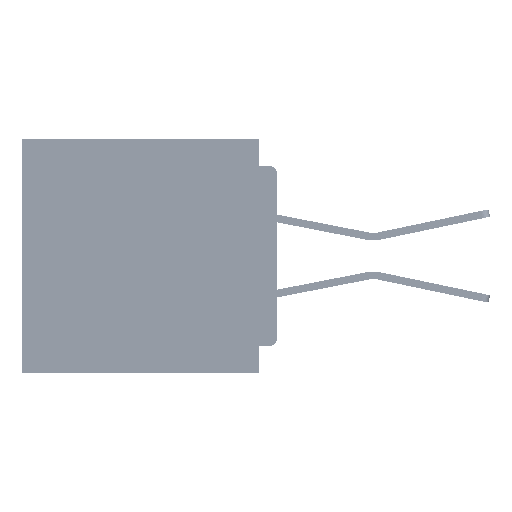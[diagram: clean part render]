
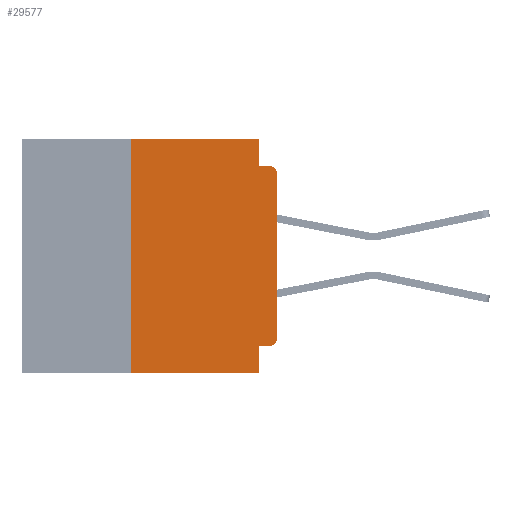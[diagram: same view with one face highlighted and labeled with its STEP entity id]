
A CAD part, left-side view. The second image highlights one B-rep face of the part: STEP entity #29577.
In plain terms, the highlighted planar face has unit normal (-1, 0, 0).
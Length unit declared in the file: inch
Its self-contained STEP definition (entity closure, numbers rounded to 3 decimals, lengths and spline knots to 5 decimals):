
#2946 = VERTEX_POINT ( 'NONE', #14960 ) ;
#3059 = EDGE_CURVE ( 'NONE', #48623, #46420, #39649, .T. ) ;
#3103 = CARTESIAN_POINT ( 'NONE',  ( 0., 0.437, 0. ) ) ;
#4556 = EDGE_CURVE ( 'NONE', #61077, #48860, #14147, .T. ) ;
#5294 = DIRECTION ( 'NONE',  ( 0., 0., -1. ) ) ;
#5375 = CARTESIAN_POINT ( 'NONE',  ( 0., 0.031, 0. ) ) ;
#5551 = VECTOR ( 'NONE', #23703, 39.37008 ) ;
#6043 = EDGE_CURVE ( 'NONE', #21826, #12576, #18952, .T. ) ;
#7128 = EDGE_CURVE ( 'NONE', #57842, #21826, #60957, .T. ) ;
#7191 = VECTOR ( 'NONE', #23229, 39.37008 ) ;
#8165 = CARTESIAN_POINT ( 'NONE',  ( 0., 0.031, -0.355 ) ) ;
#8430 = CARTESIAN_POINT ( 'NONE',  ( 0., 0.015, -0.045 ) ) ;
#8870 = EDGE_CURVE ( 'NONE', #2946, #16719, #47014, .T. ) ;
#9549 = LINE ( 'NONE', #3103, #63035 ) ;
#10191 = ORIENTED_EDGE ( 'NONE', *, *, #39013, .F. ) ;
#10314 = ORIENTED_EDGE ( 'NONE', *, *, #3059, .F. ) ;
#10898 = DIRECTION ( 'NONE',  ( -1., 0., 0. ) ) ;
#12236 = ORIENTED_EDGE ( 'NONE', *, *, #6043, .F. ) ;
#12537 = VECTOR ( 'NONE', #16501, 39.37008 ) ;
#12576 = VERTEX_POINT ( 'NONE', #44096 ) ;
#14147 = LINE ( 'NONE', #15681, #12537 ) ;
#14960 = CARTESIAN_POINT ( 'NONE',  ( 0., 0., -0.34 ) ) ;
#15681 = CARTESIAN_POINT ( 'NONE',  ( 0., 0.25, -0.4 ) ) ;
#16501 = DIRECTION ( 'NONE',  ( 0., 0., 1. ) ) ;
#16719 = VERTEX_POINT ( 'NONE', #38013 ) ;
#17970 = CARTESIAN_POINT ( 'NONE',  ( 0., 0., -0.045 ) ) ;
#18373 = ORIENTED_EDGE ( 'NONE', *, *, #56937, .T. ) ;
#18609 = VECTOR ( 'NONE', #62833, 39.37008 ) ;
#18952 = LINE ( 'NONE', #53856, #58714 ) ;
#19629 = VECTOR ( 'NONE', #37936, 39.37008 ) ;
#20200 = EDGE_CURVE ( 'NONE', #57842, #2946, #64977, .T. ) ;
#21604 = ORIENTED_EDGE ( 'NONE', *, *, #8870, .T. ) ;
#21826 = VERTEX_POINT ( 'NONE', #8165 ) ;
#21901 = CARTESIAN_POINT ( 'NONE',  ( 0., 0.437, 0. ) ) ;
#22460 = EDGE_CURVE ( 'NONE', #48860, #48623, #9549, .T. ) ;
#22821 = DIRECTION ( 'NONE',  ( 0., 0., -1. ) ) ;
#22879 = ORIENTED_EDGE ( 'NONE', *, *, #20200, .T. ) ;
#23229 = DIRECTION ( 'NONE',  ( 0., -1., 0. ) ) ;
#23473 = CARTESIAN_POINT ( 'NONE',  ( 0., 0.015, -0.06 ) ) ;
#23703 = DIRECTION ( 'NONE',  ( 0., 0., 1. ) ) ;
#27176 = DIRECTION ( 'NONE',  ( 1., 0., 0. ) ) ;
#27245 = EDGE_LOOP ( 'NONE', ( #21604, #54397, #10191, #10314, #55121, #65971, #18373, #12236, #42618, #22879 ) ) ;
#28723 = DIRECTION ( 'NONE',  ( 0., 0., -1. ) ) ;
#29577 = ADVANCED_FACE ( 'NONE', ( #39276 ), #52945, .F. ) ;
#29750 = EDGE_CURVE ( 'NONE', #16719, #57234, #40034, .T. ) ;
#31935 = CARTESIAN_POINT ( 'NONE',  ( 0., 0.437, -0.4 ) ) ;
#32375 = AXIS2_PLACEMENT_3D ( 'NONE', #23473, #59685, #28723 ) ;
#34122 = LINE ( 'NONE', #31935, #18609 ) ;
#34857 = CARTESIAN_POINT ( 'NONE',  ( 0., 0.015, -0.355 ) ) ;
#34883 = LINE ( 'NONE', #17970, #7191 ) ;
#36410 = VECTOR ( 'NONE', #5294, 39.37008 ) ;
#37928 = CARTESIAN_POINT ( 'NONE',  ( 0., 0.25, 0. ) ) ;
#37936 = DIRECTION ( 'NONE',  ( 0., 1., 0. ) ) ;
#38013 = CARTESIAN_POINT ( 'NONE',  ( 0., 0., -0.06 ) ) ;
#39013 = EDGE_CURVE ( 'NONE', #46420, #57234, #34883, .T. ) ;
#39276 = FACE_OUTER_BOUND ( 'NONE', #27245, .T. ) ;
#39649 = LINE ( 'NONE', #5375, #36410 ) ;
#40034 = CIRCLE ( 'NONE', #32375, 0.015 ) ;
#42064 = CARTESIAN_POINT ( 'NONE',  ( 0., 0.015, -0.34 ) ) ;
#42618 = ORIENTED_EDGE ( 'NONE', *, *, #7128, .F. ) ;
#43139 = CARTESIAN_POINT ( 'NONE',  ( 0., 0., -0.355 ) ) ;
#43917 = CARTESIAN_POINT ( 'NONE',  ( 0., 0.25, -0.4 ) ) ;
#44096 = CARTESIAN_POINT ( 'NONE',  ( 0., 0.031, -0.4 ) ) ;
#46420 = VERTEX_POINT ( 'NONE', #63295 ) ;
#47014 = LINE ( 'NONE', #64828, #5551 ) ;
#47242 = DIRECTION ( 'NONE',  ( 0., 0., -1. ) ) ;
#48623 = VERTEX_POINT ( 'NONE', #51316 ) ;
#48860 = VERTEX_POINT ( 'NONE', #37928 ) ;
#51316 = CARTESIAN_POINT ( 'NONE',  ( 0., 0.031, 0. ) ) ;
#52945 = PLANE ( 'NONE',  #64759 ) ;
#53856 = CARTESIAN_POINT ( 'NONE',  ( 0., 0.031, -0.4 ) ) ;
#54397 = ORIENTED_EDGE ( 'NONE', *, *, #29750, .T. ) ;
#55121 = ORIENTED_EDGE ( 'NONE', *, *, #22460, .F. ) ;
#56937 = EDGE_CURVE ( 'NONE', #61077, #12576, #34122, .T. ) ;
#57234 = VERTEX_POINT ( 'NONE', #8430 ) ;
#57842 = VERTEX_POINT ( 'NONE', #34857 ) ;
#58714 = VECTOR ( 'NONE', #22821, 39.37008 ) ;
#59685 = DIRECTION ( 'NONE',  ( -1., 0., 0. ) ) ;
#60224 = DIRECTION ( 'NONE',  ( 0., -1., 0. ) ) ;
#60957 = LINE ( 'NONE', #43139, #19629 ) ;
#61077 = VERTEX_POINT ( 'NONE', #43917 ) ;
#62833 = DIRECTION ( 'NONE',  ( 0., -1., 0. ) ) ;
#63035 = VECTOR ( 'NONE', #60224, 39.37008 ) ;
#63288 = DIRECTION ( 'NONE',  ( 0., 0., -1. ) ) ;
#63295 = CARTESIAN_POINT ( 'NONE',  ( 0., 0.031, -0.045 ) ) ;
#64532 = AXIS2_PLACEMENT_3D ( 'NONE', #42064, #10898, #47242 ) ;
#64759 = AXIS2_PLACEMENT_3D ( 'NONE', #21901, #27176, #63288 ) ;
#64828 = CARTESIAN_POINT ( 'NONE',  ( 0., 0., 0. ) ) ;
#64977 = CIRCLE ( 'NONE', #64532, 0.015 ) ;
#65971 = ORIENTED_EDGE ( 'NONE', *, *, #4556, .F. ) ;
